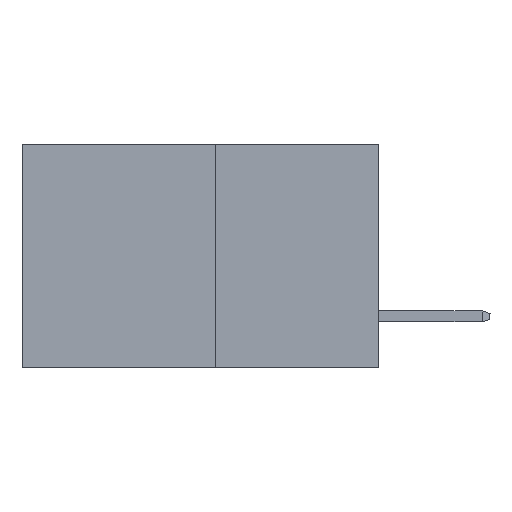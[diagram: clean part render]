
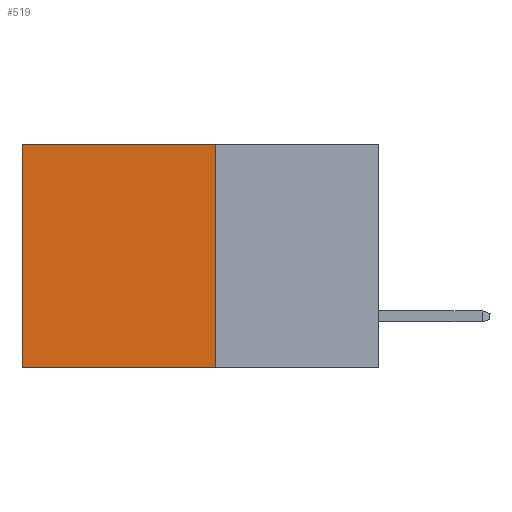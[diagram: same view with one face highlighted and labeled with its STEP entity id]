
A CAD part, left-side view. The second image highlights one B-rep face of the part: STEP entity #519.
In plain terms, the highlighted planar face has unit normal (-1, 0, 0).
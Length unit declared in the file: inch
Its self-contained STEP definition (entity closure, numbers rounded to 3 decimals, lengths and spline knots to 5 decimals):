
#320 = CARTESIAN_POINT ( 'NONE',  ( 0.277, 0.27, 0. ) ) ;
#332 = PLANE ( 'NONE',  #8245 ) ;
#335 = CARTESIAN_POINT ( 'NONE',  ( 0.277, 0.59, -0.37 ) ) ;
#519 = ADVANCED_FACE ( 'NONE', ( #8537 ), #332, .F. ) ;
#905 = DIRECTION ( 'NONE',  ( 1., 0., 0. ) ) ;
#1719 = DIRECTION ( 'NONE',  ( 0., 0., -1. ) ) ;
#3075 = EDGE_LOOP ( 'NONE', ( #6626, #12559, #8145, #9928 ) ) ;
#3299 = EDGE_CURVE ( 'NONE', #5143, #14830, #16058, .T. ) ;
#3429 = VECTOR ( 'NONE', #5119, 39.37008 ) ;
#3879 = CARTESIAN_POINT ( 'NONE',  ( 0.277, 0.27, -0.37 ) ) ;
#4051 = CARTESIAN_POINT ( 'NONE',  ( 0.277, 0.59, -0.37 ) ) ;
#4557 = EDGE_CURVE ( 'NONE', #11190, #14830, #4860, .T. ) ;
#4590 = CARTESIAN_POINT ( 'NONE',  ( 0.277, 0.59, 0. ) ) ;
#4860 = LINE ( 'NONE', #335, #10957 ) ;
#5119 = DIRECTION ( 'NONE',  ( 0., 1., 0. ) ) ;
#5142 = EDGE_CURVE ( 'NONE', #7656, #11190, #9952, .T. ) ;
#5143 = VERTEX_POINT ( 'NONE', #7880 ) ;
#5499 = DIRECTION ( 'NONE',  ( 0., 0., -1. ) ) ;
#6366 = DIRECTION ( 'NONE',  ( 0., 0., -1. ) ) ;
#6626 = ORIENTED_EDGE ( 'NONE', *, *, #4557, .T. ) ;
#6800 = VECTOR ( 'NONE', #9217, 39.37008 ) ;
#7656 = VERTEX_POINT ( 'NONE', #320 ) ;
#7880 = CARTESIAN_POINT ( 'NONE',  ( 0.277, 0.27, -0.37 ) ) ;
#7952 = LINE ( 'NONE', #3879, #14004 ) ;
#8145 = ORIENTED_EDGE ( 'NONE', *, *, #8966, .F. ) ;
#8245 = AXIS2_PLACEMENT_3D ( 'NONE', #15281, #905, #5499 ) ;
#8537 = FACE_OUTER_BOUND ( 'NONE', #3075, .T. ) ;
#8966 = EDGE_CURVE ( 'NONE', #7656, #5143, #7952, .T. ) ;
#9217 = DIRECTION ( 'NONE',  ( 0., 1., 0. ) ) ;
#9264 = CARTESIAN_POINT ( 'NONE',  ( 0.277, 0.27, -0.37 ) ) ;
#9928 = ORIENTED_EDGE ( 'NONE', *, *, #5142, .T. ) ;
#9952 = LINE ( 'NONE', #11194, #3429 ) ;
#10957 = VECTOR ( 'NONE', #1719, 39.37008 ) ;
#11190 = VERTEX_POINT ( 'NONE', #4590 ) ;
#11194 = CARTESIAN_POINT ( 'NONE',  ( 0.277, 0.27, 0. ) ) ;
#12559 = ORIENTED_EDGE ( 'NONE', *, *, #3299, .F. ) ;
#14004 = VECTOR ( 'NONE', #6366, 39.37008 ) ;
#14830 = VERTEX_POINT ( 'NONE', #4051 ) ;
#15281 = CARTESIAN_POINT ( 'NONE',  ( 0.277, 0.27, -0.37 ) ) ;
#16058 = LINE ( 'NONE', #9264, #6800 ) ;
